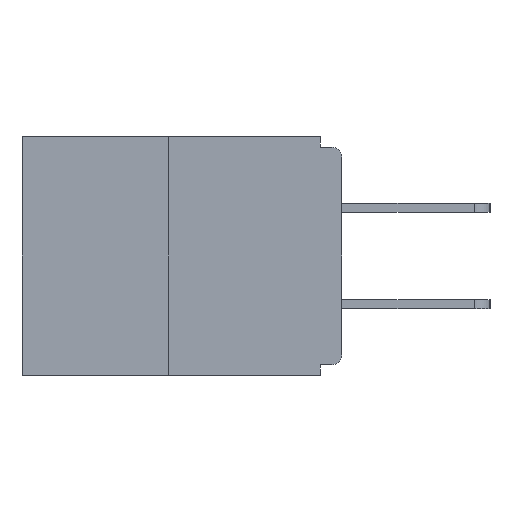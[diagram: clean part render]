
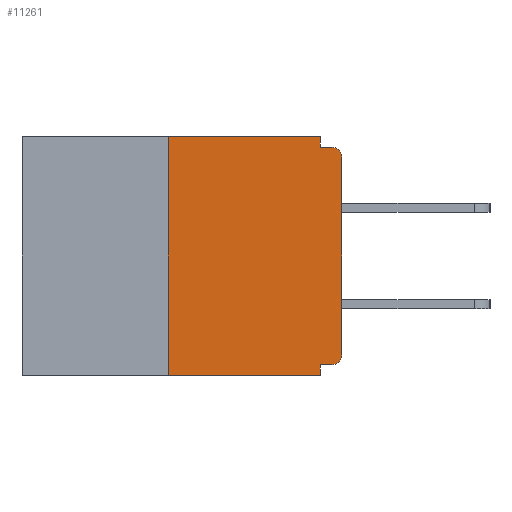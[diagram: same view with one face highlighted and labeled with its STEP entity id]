
A CAD part, left-side view. The second image highlights one B-rep face of the part: STEP entity #11261.
In plain terms, the highlighted planar face has unit normal (-1, 0, 0).
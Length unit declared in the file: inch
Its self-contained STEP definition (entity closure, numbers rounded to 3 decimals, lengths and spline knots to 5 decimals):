
#24 = DIRECTION ( 'NONE',  ( 1., 0., 0. ) ) ;
#103 = VERTEX_POINT ( 'NONE', #1495 ) ;
#122 = CARTESIAN_POINT ( 'NONE',  ( 0., 0.031, 0. ) ) ;
#278 = VERTEX_POINT ( 'NONE', #6283 ) ;
#320 = ORIENTED_EDGE ( 'NONE', *, *, #8298, .T. ) ;
#439 = ORIENTED_EDGE ( 'NONE', *, *, #2269, .T. ) ;
#613 = DIRECTION ( 'NONE',  ( 0., -1., 0. ) ) ;
#804 = DIRECTION ( 'NONE',  ( 0., 0., -1. ) ) ;
#1194 = EDGE_CURVE ( 'NONE', #11123, #3321, #2733, .T. ) ;
#1275 = CARTESIAN_POINT ( 'NONE',  ( 0., 0.25, 0. ) ) ;
#1278 = CARTESIAN_POINT ( 'NONE',  ( 0., 0., 0. ) ) ;
#1491 = EDGE_CURVE ( 'NONE', #3321, #103, #10334, .T. ) ;
#1495 = CARTESIAN_POINT ( 'NONE',  ( 0., 0.031, -0.015 ) ) ;
#1566 = FACE_OUTER_BOUND ( 'NONE', #2801, .T. ) ;
#1697 = VECTOR ( 'NONE', #5135, 39.37008 ) ;
#1925 = VERTEX_POINT ( 'NONE', #6321 ) ;
#2269 = EDGE_CURVE ( 'NONE', #1925, #11946, #4587, .T. ) ;
#2436 = DIRECTION ( 'NONE',  ( 0., -1., 0. ) ) ;
#2711 = DIRECTION ( 'NONE',  ( -1., 0., 0. ) ) ;
#2733 = LINE ( 'NONE', #7612, #4332 ) ;
#2783 = CARTESIAN_POINT ( 'NONE',  ( 0., 0.46, 0. ) ) ;
#2799 = VERTEX_POINT ( 'NONE', #8987 ) ;
#2801 = EDGE_LOOP ( 'NONE', ( #7991, #8062, #10405, #4933, #5022, #9833, #439, #320, #6333, #5979 ) ) ;
#2859 = DIRECTION ( 'NONE',  ( 0., 0., -1. ) ) ;
#3321 = VERTEX_POINT ( 'NONE', #122 ) ;
#3376 = VECTOR ( 'NONE', #613, 39.37008 ) ;
#3406 = CARTESIAN_POINT ( 'NONE',  ( 0., 0.46, -0.343 ) ) ;
#3695 = DIRECTION ( 'NONE',  ( 0., 0., -1. ) ) ;
#3999 = VECTOR ( 'NONE', #5491, 39.37008 ) ;
#4149 = CARTESIAN_POINT ( 'NONE',  ( 0., 0.015, -0.313 ) ) ;
#4232 = CARTESIAN_POINT ( 'NONE',  ( 0., 0.015, -0.015 ) ) ;
#4332 = VECTOR ( 'NONE', #9536, 39.37008 ) ;
#4548 = CIRCLE ( 'NONE', #5477, 0.015 ) ;
#4587 = LINE ( 'NONE', #1278, #6485 ) ;
#4616 = LINE ( 'NONE', #5223, #1697 ) ;
#4720 = EDGE_CURVE ( 'NONE', #2799, #10457, #4616, .T. ) ;
#4933 = ORIENTED_EDGE ( 'NONE', *, *, #5999, .F. ) ;
#5004 = VECTOR ( 'NONE', #7832, 39.37008 ) ;
#5022 = ORIENTED_EDGE ( 'NONE', *, *, #4720, .F. ) ;
#5077 = DIRECTION ( 'NONE',  ( 0., 0., -1. ) ) ;
#5135 = DIRECTION ( 'NONE',  ( 0., 1., 0. ) ) ;
#5223 = CARTESIAN_POINT ( 'NONE',  ( 0., 0., -0.328 ) ) ;
#5266 = LINE ( 'NONE', #3406, #3376 ) ;
#5477 = AXIS2_PLACEMENT_3D ( 'NONE', #8312, #2711, #3695 ) ;
#5491 = DIRECTION ( 'NONE',  ( 0., 0., -1. ) ) ;
#5506 = VECTOR ( 'NONE', #2436, 39.37008 ) ;
#5594 = VERTEX_POINT ( 'NONE', #11428 ) ;
#5610 = CARTESIAN_POINT ( 'NONE',  ( 0., 0., -0.03 ) ) ;
#5624 = PLANE ( 'NONE',  #10521 ) ;
#5646 = LINE ( 'NONE', #9041, #5506 ) ;
#5979 = ORIENTED_EDGE ( 'NONE', *, *, #1491, .F. ) ;
#5999 = EDGE_CURVE ( 'NONE', #10457, #5594, #7368, .T. ) ;
#6283 = CARTESIAN_POINT ( 'NONE',  ( 0., 0.25, -0.343 ) ) ;
#6321 = CARTESIAN_POINT ( 'NONE',  ( 0., 0., -0.313 ) ) ;
#6333 = ORIENTED_EDGE ( 'NONE', *, *, #11668, .F. ) ;
#6485 = VECTOR ( 'NONE', #9910, 39.37008 ) ;
#7181 = CARTESIAN_POINT ( 'NONE',  ( 0., 0.031, -0.343 ) ) ;
#7362 = EDGE_CURVE ( 'NONE', #2799, #1925, #8805, .T. ) ;
#7368 = LINE ( 'NONE', #7181, #3999 ) ;
#7612 = CARTESIAN_POINT ( 'NONE',  ( 0., 0.46, 0. ) ) ;
#7832 = DIRECTION ( 'NONE',  ( 0., 0., 1. ) ) ;
#7991 = ORIENTED_EDGE ( 'NONE', *, *, #1194, .F. ) ;
#8062 = ORIENTED_EDGE ( 'NONE', *, *, #9197, .F. ) ;
#8207 = EDGE_CURVE ( 'NONE', #278, #5594, #5266, .T. ) ;
#8220 = CARTESIAN_POINT ( 'NONE',  ( 0., 0.031, 0. ) ) ;
#8298 = EDGE_CURVE ( 'NONE', #11946, #9330, #4548, .T. ) ;
#8303 = AXIS2_PLACEMENT_3D ( 'NONE', #4149, #10731, #5077 ) ;
#8312 = CARTESIAN_POINT ( 'NONE',  ( 0., 0.015, -0.03 ) ) ;
#8805 = CIRCLE ( 'NONE', #8303, 0.015 ) ;
#8929 = LINE ( 'NONE', #1275, #5004 ) ;
#8987 = CARTESIAN_POINT ( 'NONE',  ( 0., 0.015, -0.328 ) ) ;
#9041 = CARTESIAN_POINT ( 'NONE',  ( 0., 0., -0.015 ) ) ;
#9197 = EDGE_CURVE ( 'NONE', #278, #11123, #8929, .T. ) ;
#9330 = VERTEX_POINT ( 'NONE', #4232 ) ;
#9536 = DIRECTION ( 'NONE',  ( 0., -1., 0. ) ) ;
#9833 = ORIENTED_EDGE ( 'NONE', *, *, #7362, .T. ) ;
#9910 = DIRECTION ( 'NONE',  ( 0., 0., 1. ) ) ;
#9969 = CARTESIAN_POINT ( 'NONE',  ( 0., 0.031, -0.328 ) ) ;
#10334 = LINE ( 'NONE', #8220, #11485 ) ;
#10405 = ORIENTED_EDGE ( 'NONE', *, *, #8207, .T. ) ;
#10457 = VERTEX_POINT ( 'NONE', #9969 ) ;
#10521 = AXIS2_PLACEMENT_3D ( 'NONE', #2783, #24, #2859 ) ;
#10731 = DIRECTION ( 'NONE',  ( -1., 0., 0. ) ) ;
#10954 = CARTESIAN_POINT ( 'NONE',  ( 0., 0.25, 0. ) ) ;
#11123 = VERTEX_POINT ( 'NONE', #10954 ) ;
#11261 = ADVANCED_FACE ( 'NONE', ( #1566 ), #5624, .F. ) ;
#11428 = CARTESIAN_POINT ( 'NONE',  ( 0., 0.031, -0.343 ) ) ;
#11485 = VECTOR ( 'NONE', #804, 39.37008 ) ;
#11668 = EDGE_CURVE ( 'NONE', #103, #9330, #5646, .T. ) ;
#11946 = VERTEX_POINT ( 'NONE', #5610 ) ;
